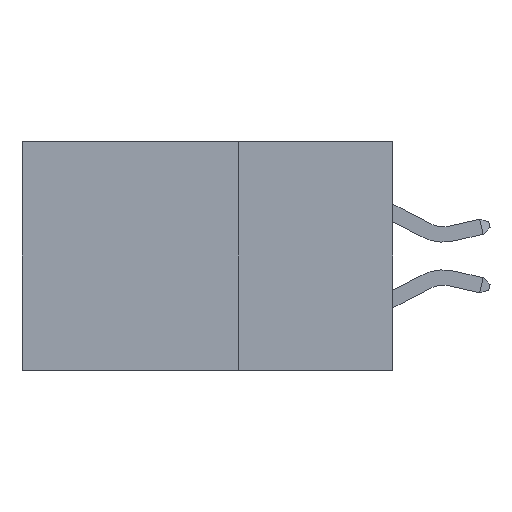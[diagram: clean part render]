
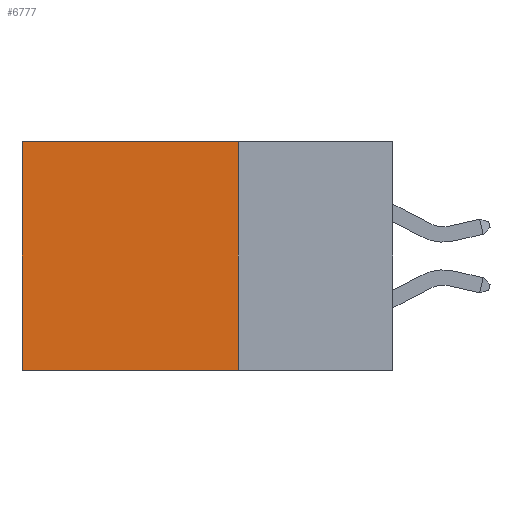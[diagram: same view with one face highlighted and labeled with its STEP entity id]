
A CAD part, left-side view. The second image highlights one B-rep face of the part: STEP entity #6777.
In plain terms, the highlighted planar face has unit normal (-1, 0, 0).
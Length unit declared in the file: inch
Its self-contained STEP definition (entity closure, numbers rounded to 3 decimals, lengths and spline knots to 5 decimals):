
#628 = LINE ( 'NONE', #6419, #22620 ) ;
#1148 = EDGE_CURVE ( 'NONE', #24795, #19483, #628, .T. ) ;
#1604 = ORIENTED_EDGE ( 'NONE', *, *, #12373, .F. ) ;
#5040 = PLANE ( 'NONE',  #15666 ) ;
#6057 = DIRECTION ( 'NONE',  ( 0., 0., -1. ) ) ;
#6359 = CARTESIAN_POINT ( 'NONE',  ( 0.2875, 0.25, 0. ) ) ;
#6419 = CARTESIAN_POINT ( 'NONE',  ( 0.2875, 0.6, 0. ) ) ;
#6559 = CARTESIAN_POINT ( 'NONE',  ( 0.2875, 0.6, -0.37 ) ) ;
#6662 = ORIENTED_EDGE ( 'NONE', *, *, #1148, .T. ) ;
#6777 = ADVANCED_FACE ( 'NONE', ( #20742 ), #5040, .F. ) ;
#7469 = LINE ( 'NONE', #23903, #23716 ) ;
#7623 = CARTESIAN_POINT ( 'NONE',  ( 0.2875, 0.25, -0.37 ) ) ;
#8563 = EDGE_CURVE ( 'NONE', #10505, #24795, #15701, .T. ) ;
#9111 = CARTESIAN_POINT ( 'NONE',  ( 0.2875, 0.25, 0. ) ) ;
#10029 = VECTOR ( 'NONE', #19634, 39.37008 ) ;
#10505 = VERTEX_POINT ( 'NONE', #9111 ) ;
#11058 = LINE ( 'NONE', #11280, #20992 ) ;
#11280 = CARTESIAN_POINT ( 'NONE',  ( 0.2875, 0.25, 0. ) ) ;
#11513 = CARTESIAN_POINT ( 'NONE',  ( 0.2875, 0.25, 0. ) ) ;
#12373 = EDGE_CURVE ( 'NONE', #13834, #19483, #7469, .T. ) ;
#13656 = DIRECTION ( 'NONE',  ( 0., 0., -1. ) ) ;
#13834 = VERTEX_POINT ( 'NONE', #7623 ) ;
#14230 = EDGE_LOOP ( 'NONE', ( #6662, #1604, #17384, #16373 ) ) ;
#15666 = AXIS2_PLACEMENT_3D ( 'NONE', #11513, #26165, #13656 ) ;
#15701 = LINE ( 'NONE', #6359, #10029 ) ;
#16373 = ORIENTED_EDGE ( 'NONE', *, *, #8563, .T. ) ;
#16945 = EDGE_CURVE ( 'NONE', #10505, #13834, #11058, .T. ) ;
#17384 = ORIENTED_EDGE ( 'NONE', *, *, #16945, .F. ) ;
#17714 = DIRECTION ( 'NONE',  ( 0., 0., -1. ) ) ;
#19483 = VERTEX_POINT ( 'NONE', #6559 ) ;
#19634 = DIRECTION ( 'NONE',  ( 0., 1., 0. ) ) ;
#19733 = DIRECTION ( 'NONE',  ( 0., 1., 0. ) ) ;
#20742 = FACE_OUTER_BOUND ( 'NONE', #14230, .T. ) ;
#20992 = VECTOR ( 'NONE', #17714, 39.37008 ) ;
#22620 = VECTOR ( 'NONE', #6057, 39.37008 ) ;
#23716 = VECTOR ( 'NONE', #19733, 39.37008 ) ;
#23903 = CARTESIAN_POINT ( 'NONE',  ( 0.2875, 0.25, -0.37 ) ) ;
#24795 = VERTEX_POINT ( 'NONE', #24952 ) ;
#24952 = CARTESIAN_POINT ( 'NONE',  ( 0.2875, 0.6, 0. ) ) ;
#26165 = DIRECTION ( 'NONE',  ( 1., 0., 0. ) ) ;
